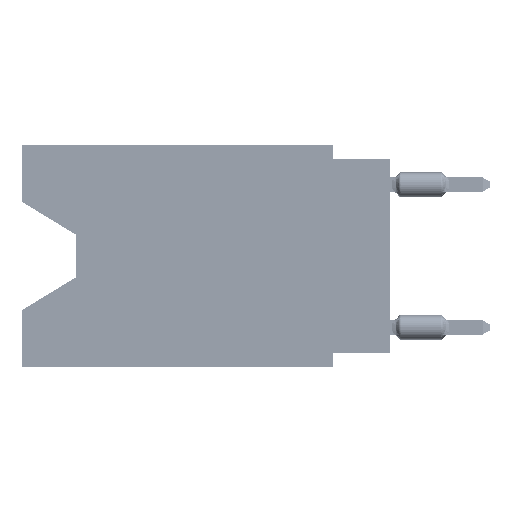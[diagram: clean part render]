
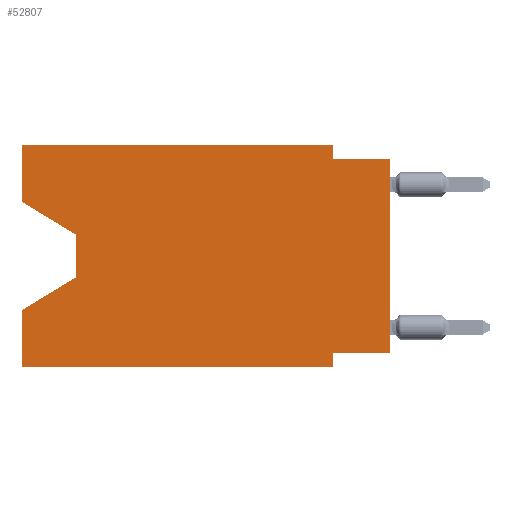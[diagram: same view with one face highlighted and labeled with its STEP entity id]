
A CAD part, left-side view. The second image highlights one B-rep face of the part: STEP entity #52807.
In plain terms, the highlighted planar face has unit normal (-1, 0, 0).
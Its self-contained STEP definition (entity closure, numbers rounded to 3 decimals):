
#210 = DIRECTION ( 'NONE',  ( 0., 0., -1. ) ) ;
#844 = ORIENTED_EDGE ( 'NONE', *, *, #36370, .T. ) ;
#3135 = DIRECTION ( 'NONE',  ( 0., -1., 0. ) ) ;
#5928 = ORIENTED_EDGE ( 'NONE', *, *, #64466, .F. ) ;
#6315 = DIRECTION ( 'NONE',  ( 0., 0.855, -0.519 ) ) ;
#6707 = EDGE_CURVE ( 'NONE', #28554, #34549, #50967, .T. ) ;
#7001 = PLANE ( 'NONE',  #31972 ) ;
#7722 = CARTESIAN_POINT ( 'NONE',  ( 0., 13.97, -4.013 ) ) ;
#8539 = DIRECTION ( 'NONE',  ( 0., -0.855, -0.519 ) ) ;
#10239 = CARTESIAN_POINT ( 'NONE',  ( 0., 16.383, 0. ) ) ;
#11149 = LINE ( 'NONE', #16822, #16888 ) ;
#11412 = CARTESIAN_POINT ( 'NONE',  ( 0., 16.383, -9.906 ) ) ;
#12133 = VECTOR ( 'NONE', #69534, 1000. ) ;
#12195 = CARTESIAN_POINT ( 'NONE',  ( 0., 0., -9.271 ) ) ;
#12722 = EDGE_CURVE ( 'NONE', #17303, #36081, #27958, .T. ) ;
#13305 = VERTEX_POINT ( 'NONE', #24360 ) ;
#13350 = LINE ( 'NONE', #43537, #24116 ) ;
#13808 = EDGE_CURVE ( 'NONE', #13305, #19250, #63927, .T. ) ;
#14067 = VECTOR ( 'NONE', #8539, 1000. ) ;
#14386 = CARTESIAN_POINT ( 'NONE',  ( 0., 0., -0.635 ) ) ;
#15198 = CARTESIAN_POINT ( 'NONE',  ( 0., 16.383, -9.906 ) ) ;
#16338 = ORIENTED_EDGE ( 'NONE', *, *, #48827, .F. ) ;
#16822 = CARTESIAN_POINT ( 'NONE',  ( 0., 2.54, 0. ) ) ;
#16888 = VECTOR ( 'NONE', #69285, 1000. ) ;
#17303 = VERTEX_POINT ( 'NONE', #74057 ) ;
#18695 = VERTEX_POINT ( 'NONE', #19675 ) ;
#19250 = VERTEX_POINT ( 'NONE', #20336 ) ;
#19675 = CARTESIAN_POINT ( 'NONE',  ( 0., 2.54, -9.906 ) ) ;
#19917 = CARTESIAN_POINT ( 'NONE',  ( 0., 2.54, -0.635 ) ) ;
#19951 = VERTEX_POINT ( 'NONE', #43466 ) ;
#20336 = CARTESIAN_POINT ( 'NONE',  ( 0., 2.54, -9.271 ) ) ;
#20994 = CARTESIAN_POINT ( 'NONE',  ( 0., 16.383, -2.546 ) ) ;
#21689 = CARTESIAN_POINT ( 'NONE',  ( 0., 2.54, -9.906 ) ) ;
#23453 = LINE ( 'NONE', #46485, #12133 ) ;
#23825 = LINE ( 'NONE', #70640, #35178 ) ;
#23950 = VERTEX_POINT ( 'NONE', #14386 ) ;
#24116 = VECTOR ( 'NONE', #3135, 1000. ) ;
#24360 = CARTESIAN_POINT ( 'NONE',  ( 0., 0., -9.271 ) ) ;
#25559 = VERTEX_POINT ( 'NONE', #61507 ) ;
#25941 = ORIENTED_EDGE ( 'NONE', *, *, #46096, .F. ) ;
#26252 = EDGE_CURVE ( 'NONE', #25559, #34549, #35007, .T. ) ;
#26571 = EDGE_CURVE ( 'NONE', #36081, #56894, #11149, .T. ) ;
#27229 = ORIENTED_EDGE ( 'NONE', *, *, #6707, .F. ) ;
#27894 = VECTOR ( 'NONE', #41225, 1000. ) ;
#27958 = LINE ( 'NONE', #10239, #73230 ) ;
#28326 = DIRECTION ( 'NONE',  ( 0., -1., 0. ) ) ;
#28376 = CARTESIAN_POINT ( 'NONE',  ( 0., 13.97, -4.013 ) ) ;
#28554 = VERTEX_POINT ( 'NONE', #15198 ) ;
#30029 = CARTESIAN_POINT ( 'NONE',  ( 0., 16.383, 0. ) ) ;
#30977 = ORIENTED_EDGE ( 'NONE', *, *, #41283, .T. ) ;
#31972 = AXIS2_PLACEMENT_3D ( 'NONE', #30029, #53059, #210 ) ;
#34549 = VERTEX_POINT ( 'NONE', #52437 ) ;
#35007 = LINE ( 'NONE', #58042, #39713 ) ;
#35178 = VECTOR ( 'NONE', #64960, 1000. ) ;
#36081 = VERTEX_POINT ( 'NONE', #56912 ) ;
#36370 = EDGE_CURVE ( 'NONE', #19951, #51614, #53852, .T. ) ;
#37291 = ORIENTED_EDGE ( 'NONE', *, *, #26571, .F. ) ;
#37345 = ORIENTED_EDGE ( 'NONE', *, *, #26252, .T. ) ;
#38618 = ORIENTED_EDGE ( 'NONE', *, *, #69888, .T. ) ;
#39713 = VECTOR ( 'NONE', #6315, 1000. ) ;
#39755 = EDGE_CURVE ( 'NONE', #51614, #25559, #57086, .T. ) ;
#40041 = ORIENTED_EDGE ( 'NONE', *, *, #13808, .F. ) ;
#41225 = DIRECTION ( 'NONE',  ( 0., -1., 0. ) ) ;
#41283 = EDGE_CURVE ( 'NONE', #13305, #23950, #23825, .T. ) ;
#41956 = DIRECTION ( 'NONE',  ( 0., 0., -1. ) ) ;
#43466 = CARTESIAN_POINT ( 'NONE',  ( 0., 16.383, -2.546 ) ) ;
#43537 = CARTESIAN_POINT ( 'NONE',  ( 0., 0., -0.635 ) ) ;
#45306 = DIRECTION ( 'NONE',  ( 0., 0., 1. ) ) ;
#45404 = LINE ( 'NONE', #11412, #27894 ) ;
#46096 = EDGE_CURVE ( 'NONE', #19250, #18695, #61354, .T. ) ;
#46485 = CARTESIAN_POINT ( 'NONE',  ( 0., 16.383, 0. ) ) ;
#48169 = VECTOR ( 'NONE', #73791, 1000. ) ;
#48827 = EDGE_CURVE ( 'NONE', #56894, #23950, #13350, .T. ) ;
#50753 = EDGE_LOOP ( 'NONE', ( #844, #54038, #37345, #27229, #38618, #25941, #40041, #30977, #16338, #37291, #56853, #5928 ) ) ;
#50967 = LINE ( 'NONE', #74015, #67947 ) ;
#51614 = VERTEX_POINT ( 'NONE', #7722 ) ;
#52437 = CARTESIAN_POINT ( 'NONE',  ( 0., 16.383, -7.36 ) ) ;
#52807 = ADVANCED_FACE ( 'NONE', ( #58747 ), #7001, .F. ) ;
#53059 = DIRECTION ( 'NONE',  ( 1., 0., 0. ) ) ;
#53852 = LINE ( 'NONE', #20994, #14067 ) ;
#54038 = ORIENTED_EDGE ( 'NONE', *, *, #39755, .T. ) ;
#56698 = VECTOR ( 'NONE', #41956, 1000. ) ;
#56853 = ORIENTED_EDGE ( 'NONE', *, *, #12722, .F. ) ;
#56894 = VERTEX_POINT ( 'NONE', #19917 ) ;
#56912 = CARTESIAN_POINT ( 'NONE',  ( 0., 2.54, 0. ) ) ;
#57086 = LINE ( 'NONE', #28376, #56698 ) ;
#58042 = CARTESIAN_POINT ( 'NONE',  ( 0., 13.97, -5.893 ) ) ;
#58264 = DIRECTION ( 'NONE',  ( 0., 1., 0. ) ) ;
#58747 = FACE_OUTER_BOUND ( 'NONE', #50753, .T. ) ;
#61354 = LINE ( 'NONE', #21689, #48169 ) ;
#61507 = CARTESIAN_POINT ( 'NONE',  ( 0., 13.97, -5.893 ) ) ;
#61622 = VECTOR ( 'NONE', #58264, 1000. ) ;
#63927 = LINE ( 'NONE', #12195, #61622 ) ;
#64466 = EDGE_CURVE ( 'NONE', #19951, #17303, #23453, .T. ) ;
#64960 = DIRECTION ( 'NONE',  ( 0., 0., 1. ) ) ;
#67947 = VECTOR ( 'NONE', #45306, 1000. ) ;
#69285 = DIRECTION ( 'NONE',  ( 0., 0., -1. ) ) ;
#69534 = DIRECTION ( 'NONE',  ( 0., 0., 1. ) ) ;
#69888 = EDGE_CURVE ( 'NONE', #28554, #18695, #45404, .T. ) ;
#70640 = CARTESIAN_POINT ( 'NONE',  ( 0., 0., 0. ) ) ;
#73230 = VECTOR ( 'NONE', #28326, 1000. ) ;
#73791 = DIRECTION ( 'NONE',  ( 0., 0., -1. ) ) ;
#74015 = CARTESIAN_POINT ( 'NONE',  ( 0., 16.383, 0. ) ) ;
#74057 = CARTESIAN_POINT ( 'NONE',  ( 0., 16.383, 0. ) ) ;
